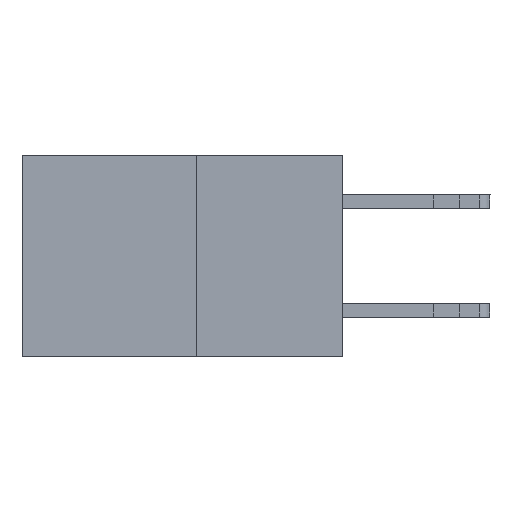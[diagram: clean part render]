
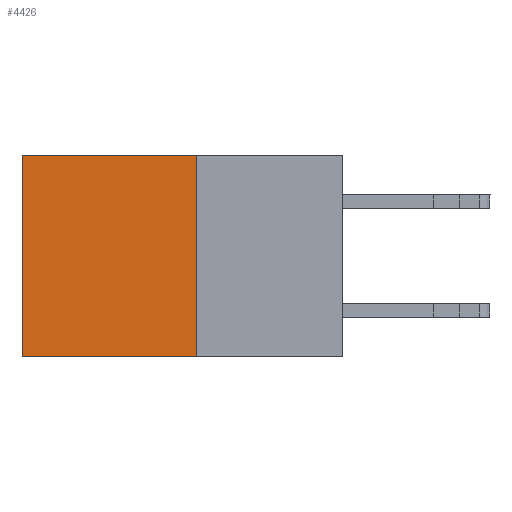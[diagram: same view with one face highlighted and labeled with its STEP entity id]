
A CAD part, left-side view. The second image highlights one B-rep face of the part: STEP entity #4426.
In plain terms, the highlighted planar face has unit normal (-1, 0, 0).
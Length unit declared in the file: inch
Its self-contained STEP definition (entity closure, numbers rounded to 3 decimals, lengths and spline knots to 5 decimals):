
#476 = CARTESIAN_POINT ( 'NONE',  ( 0.277, 0.27, 0. ) ) ;
#564 = DIRECTION ( 'NONE',  ( 0., 1., 0. ) ) ;
#692 = ORIENTED_EDGE ( 'NONE', *, *, #3970, .F. ) ;
#1094 = EDGE_CURVE ( 'NONE', #9533, #12285, #7461, .T. ) ;
#1726 = CARTESIAN_POINT ( 'NONE',  ( 0.277, 0.27, -0.37 ) ) ;
#1924 = CARTESIAN_POINT ( 'NONE',  ( 0.277, 0.27, 0. ) ) ;
#3134 = EDGE_LOOP ( 'NONE', ( #4283, #12337, #692, #13262 ) ) ;
#3399 = CARTESIAN_POINT ( 'NONE',  ( 0.277, 0.59, 0. ) ) ;
#3970 = EDGE_CURVE ( 'NONE', #9533, #16175, #11478, .T. ) ;
#4283 = ORIENTED_EDGE ( 'NONE', *, *, #17183, .T. ) ;
#4426 = ADVANCED_FACE ( 'NONE', ( #7482 ), #13223, .F. ) ;
#4625 = AXIS2_PLACEMENT_3D ( 'NONE', #16522, #15937, #16590 ) ;
#6047 = EDGE_CURVE ( 'NONE', #16175, #18606, #10242, .T. ) ;
#6959 = VECTOR ( 'NONE', #564, 39.37008 ) ;
#7209 = CARTESIAN_POINT ( 'NONE',  ( 0.277, 0.59, -0.37 ) ) ;
#7461 = LINE ( 'NONE', #476, #6959 ) ;
#7482 = FACE_OUTER_BOUND ( 'NONE', #3134, .T. ) ;
#9271 = VECTOR ( 'NONE', #13012, 39.37008 ) ;
#9533 = VERTEX_POINT ( 'NONE', #1924 ) ;
#10024 = CARTESIAN_POINT ( 'NONE',  ( 0.277, 0.59, -0.37 ) ) ;
#10242 = LINE ( 'NONE', #15191, #18251 ) ;
#11478 = LINE ( 'NONE', #1726, #19043 ) ;
#12285 = VERTEX_POINT ( 'NONE', #3399 ) ;
#12337 = ORIENTED_EDGE ( 'NONE', *, *, #6047, .F. ) ;
#13012 = DIRECTION ( 'NONE',  ( 0., 0., -1. ) ) ;
#13223 = PLANE ( 'NONE',  #4625 ) ;
#13262 = ORIENTED_EDGE ( 'NONE', *, *, #1094, .T. ) ;
#15159 = DIRECTION ( 'NONE',  ( 0., 0., -1. ) ) ;
#15191 = CARTESIAN_POINT ( 'NONE',  ( 0.277, 0.27, -0.37 ) ) ;
#15417 = DIRECTION ( 'NONE',  ( 0., 1., 0. ) ) ;
#15937 = DIRECTION ( 'NONE',  ( 1., 0., 0. ) ) ;
#16175 = VERTEX_POINT ( 'NONE', #18288 ) ;
#16522 = CARTESIAN_POINT ( 'NONE',  ( 0.277, 0.27, -0.37 ) ) ;
#16590 = DIRECTION ( 'NONE',  ( 0., 0., -1. ) ) ;
#17183 = EDGE_CURVE ( 'NONE', #12285, #18606, #17244, .T. ) ;
#17244 = LINE ( 'NONE', #10024, #9271 ) ;
#18251 = VECTOR ( 'NONE', #15417, 39.37008 ) ;
#18288 = CARTESIAN_POINT ( 'NONE',  ( 0.277, 0.27, -0.37 ) ) ;
#18606 = VERTEX_POINT ( 'NONE', #7209 ) ;
#19043 = VECTOR ( 'NONE', #15159, 39.37008 ) ;
